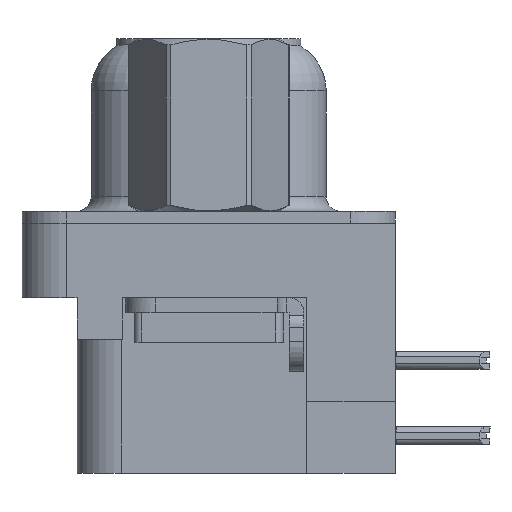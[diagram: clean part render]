
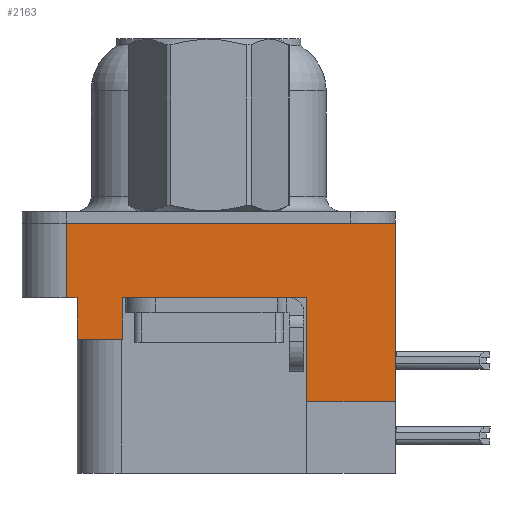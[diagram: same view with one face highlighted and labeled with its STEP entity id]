
A CAD part, left-side view. The second image highlights one B-rep face of the part: STEP entity #2163.
In plain terms, the highlighted planar face has unit normal (-1, 0, 0).
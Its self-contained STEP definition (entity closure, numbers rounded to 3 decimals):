
#136 = VERTEX_POINT ( 'NONE', #27553 ) ;
#1427 = EDGE_CURVE ( 'NONE', #4689, #8168, #18745, .T. ) ;
#1595 = ORIENTED_EDGE ( 'NONE', *, *, #1427, .T. ) ;
#1650 = ORIENTED_EDGE ( 'NONE', *, *, #2697, .F. ) ;
#2163 = ADVANCED_FACE ( 'NONE', ( #13899 ), #12527, .T. ) ;
#2432 = CARTESIAN_POINT ( 'NONE',  ( -2.935, -3.295, -8.4 ) ) ;
#2697 = EDGE_CURVE ( 'NONE', #4689, #17473, #18681, .T. ) ;
#2954 = DIRECTION ( 'NONE',  ( 0., -1., 0. ) ) ;
#3140 = LINE ( 'NONE', #28007, #21277 ) ;
#3689 = DIRECTION ( 'NONE',  ( 0., 0., 1. ) ) ;
#3785 = CARTESIAN_POINT ( 'NONE',  ( -2.935, -3.295, -6. ) ) ;
#4039 = EDGE_CURVE ( 'NONE', #14803, #5284, #6576, .T. ) ;
#4689 = VERTEX_POINT ( 'NONE', #29529 ) ;
#4781 = LINE ( 'NONE', #4841, #22143 ) ;
#4841 = CARTESIAN_POINT ( 'NONE',  ( -2.935, 4.425, -3.9 ) ) ;
#5223 = ORIENTED_EDGE ( 'NONE', *, *, #4039, .F. ) ;
#5284 = VERTEX_POINT ( 'NONE', #22704 ) ;
#5285 = CARTESIAN_POINT ( 'NONE',  ( -2.935, 4.425, -2.5 ) ) ;
#5661 = AXIS2_PLACEMENT_3D ( 'NONE', #21709, #10688, #3689 ) ;
#5998 = CARTESIAN_POINT ( 'NONE',  ( -2.935, 2.895, -3.9 ) ) ;
#6165 = VECTOR ( 'NONE', #2954, 1000. ) ;
#6576 = LINE ( 'NONE', #2432, #12125 ) ;
#6602 = LINE ( 'NONE', #20084, #30233 ) ;
#7796 = CARTESIAN_POINT ( 'NONE',  ( -2.935, 4.775, -2.5 ) ) ;
#8168 = VERTEX_POINT ( 'NONE', #5285 ) ;
#8662 = VERTEX_POINT ( 'NONE', #20871 ) ;
#9601 = DIRECTION ( 'NONE',  ( 0., 1., 0. ) ) ;
#10313 = VECTOR ( 'NONE', #20169, 1000. ) ;
#10688 = DIRECTION ( 'NONE',  ( -1., 0., 0. ) ) ;
#10808 = EDGE_LOOP ( 'NONE', ( #28469, #25934, #14172, #1650, #1595, #11758, #15430, #25122, #20832, #5223 ) ) ;
#11054 = LINE ( 'NONE', #5998, #10313 ) ;
#11758 = ORIENTED_EDGE ( 'NONE', *, *, #23130, .F. ) ;
#12125 = VECTOR ( 'NONE', #18978, 1000. ) ;
#12527 = PLANE ( 'NONE',  #5661 ) ;
#12546 = EDGE_CURVE ( 'NONE', #23407, #8662, #4781, .T. ) ;
#12752 = VECTOR ( 'NONE', #26042, 1000. ) ;
#12803 = VERTEX_POINT ( 'NONE', #26532 ) ;
#13835 = CARTESIAN_POINT ( 'NONE',  ( -2.935, 4.775, 0. ) ) ;
#13899 = FACE_OUTER_BOUND ( 'NONE', #10808, .T. ) ;
#14172 = ORIENTED_EDGE ( 'NONE', *, *, #14498, .F. ) ;
#14498 = EDGE_CURVE ( 'NONE', #17473, #12803, #18313, .T. ) ;
#14681 = CARTESIAN_POINT ( 'NONE',  ( -2.935, -6.275, -2.5 ) ) ;
#14717 = EDGE_CURVE ( 'NONE', #136, #12803, #15334, .T. ) ;
#14803 = VERTEX_POINT ( 'NONE', #3785 ) ;
#15334 = LINE ( 'NONE', #22386, #20151 ) ;
#15430 = ORIENTED_EDGE ( 'NONE', *, *, #12546, .F. ) ;
#16211 = DIRECTION ( 'NONE',  ( 0., 0., 1. ) ) ;
#17473 = VERTEX_POINT ( 'NONE', #13835 ) ;
#17525 = EDGE_CURVE ( 'NONE', #19322, #5284, #21502, .T. ) ;
#17939 = VECTOR ( 'NONE', #23521, 1000. ) ;
#18313 = LINE ( 'NONE', #21382, #12752 ) ;
#18681 = LINE ( 'NONE', #7796, #17939 ) ;
#18745 = LINE ( 'NONE', #14681, #6165 ) ;
#18978 = DIRECTION ( 'NONE',  ( 0., 0., 1. ) ) ;
#19322 = VERTEX_POINT ( 'NONE', #27573 ) ;
#20033 = VECTOR ( 'NONE', #28180, 1000. ) ;
#20084 = CARTESIAN_POINT ( 'NONE',  ( -2.935, -6.495, -6. ) ) ;
#20151 = VECTOR ( 'NONE', #24792, 1000. ) ;
#20169 = DIRECTION ( 'NONE',  ( 0., 0., 1. ) ) ;
#20408 = EDGE_CURVE ( 'NONE', #136, #14803, #6602, .T. ) ;
#20832 = ORIENTED_EDGE ( 'NONE', *, *, #17525, .T. ) ;
#20871 = CARTESIAN_POINT ( 'NONE',  ( -2.935, 4.425, -3.9 ) ) ;
#21277 = VECTOR ( 'NONE', #16211, 1000. ) ;
#21382 = CARTESIAN_POINT ( 'NONE',  ( -2.935, -6.275, 0. ) ) ;
#21502 = LINE ( 'NONE', #28082, #20033 ) ;
#21709 = CARTESIAN_POINT ( 'NONE',  ( -2.935, -6.275, -2.5 ) ) ;
#22143 = VECTOR ( 'NONE', #9601, 1000. ) ;
#22386 = CARTESIAN_POINT ( 'NONE',  ( -2.935, -6.275, -2.5 ) ) ;
#22446 = DIRECTION ( 'NONE',  ( 0., 1., 0. ) ) ;
#22704 = CARTESIAN_POINT ( 'NONE',  ( -2.935, -3.295, -2.5 ) ) ;
#23130 = EDGE_CURVE ( 'NONE', #8662, #8168, #3140, .T. ) ;
#23407 = VERTEX_POINT ( 'NONE', #26962 ) ;
#23521 = DIRECTION ( 'NONE',  ( 0., 0., 1. ) ) ;
#24792 = DIRECTION ( 'NONE',  ( 0., 0., 1. ) ) ;
#25122 = ORIENTED_EDGE ( 'NONE', *, *, #29173, .T. ) ;
#25934 = ORIENTED_EDGE ( 'NONE', *, *, #14717, .T. ) ;
#26042 = DIRECTION ( 'NONE',  ( 0., -1., 0. ) ) ;
#26532 = CARTESIAN_POINT ( 'NONE',  ( -2.935, -6.275, 0. ) ) ;
#26962 = CARTESIAN_POINT ( 'NONE',  ( -2.935, 2.895, -3.9 ) ) ;
#27553 = CARTESIAN_POINT ( 'NONE',  ( -2.935, -6.275, -6. ) ) ;
#27573 = CARTESIAN_POINT ( 'NONE',  ( -2.935, 2.895, -2.5 ) ) ;
#28007 = CARTESIAN_POINT ( 'NONE',  ( -2.935, 4.425, -3.9 ) ) ;
#28082 = CARTESIAN_POINT ( 'NONE',  ( -2.935, -6.275, -2.5 ) ) ;
#28180 = DIRECTION ( 'NONE',  ( 0., -1., 0. ) ) ;
#28469 = ORIENTED_EDGE ( 'NONE', *, *, #20408, .F. ) ;
#29173 = EDGE_CURVE ( 'NONE', #23407, #19322, #11054, .T. ) ;
#29529 = CARTESIAN_POINT ( 'NONE',  ( -2.935, 4.775, -2.5 ) ) ;
#30233 = VECTOR ( 'NONE', #22446, 1000. ) ;
